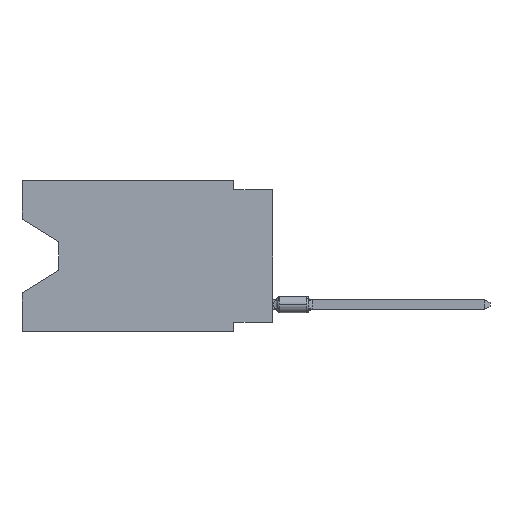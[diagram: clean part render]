
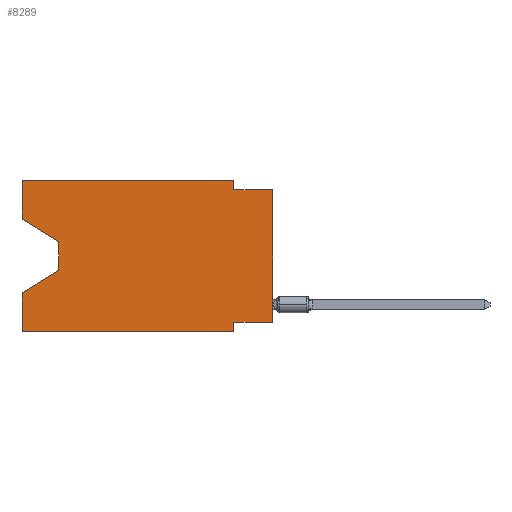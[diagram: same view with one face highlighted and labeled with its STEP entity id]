
A CAD part, left-side view. The second image highlights one B-rep face of the part: STEP entity #8289.
In plain terms, the highlighted planar face has unit normal (-1, 0, 0).
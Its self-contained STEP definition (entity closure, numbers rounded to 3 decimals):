
#38 = EDGE_CURVE ( 'NONE', #6992, #4554, #11585, .T. ) ;
#51 = CARTESIAN_POINT ( 'NONE',  ( 0., 16.383, 0. ) ) ;
#261 = ORIENTED_EDGE ( 'NONE', *, *, #5216, .T. ) ;
#657 = EDGE_CURVE ( 'NONE', #16384, #6992, #19137, .T. ) ;
#970 = CARTESIAN_POINT ( 'NONE',  ( 0., 16.383, 0. ) ) ;
#1034 = DIRECTION ( 'NONE',  ( 0., 0., -1. ) ) ;
#1234 = DIRECTION ( 'NONE',  ( 0., 0., 1. ) ) ;
#1344 = ORIENTED_EDGE ( 'NONE', *, *, #7838, .F. ) ;
#1373 = ORIENTED_EDGE ( 'NONE', *, *, #19129, .F. ) ;
#1385 = VERTEX_POINT ( 'NONE', #15082 ) ;
#1623 = CARTESIAN_POINT ( 'NONE',  ( 0., 13.97, -5.893 ) ) ;
#1732 = DIRECTION ( 'NONE',  ( 0., 0., -1. ) ) ;
#1779 = LINE ( 'NONE', #13912, #6685 ) ;
#2070 = VERTEX_POINT ( 'NONE', #4231 ) ;
#2116 = ORIENTED_EDGE ( 'NONE', *, *, #10446, .T. ) ;
#2195 = CARTESIAN_POINT ( 'NONE',  ( 0., 2.54, -0.635 ) ) ;
#2518 = VECTOR ( 'NONE', #7438, 1000. ) ;
#2958 = EDGE_CURVE ( 'NONE', #16225, #16384, #17965, .T. ) ;
#3040 = CARTESIAN_POINT ( 'NONE',  ( 0., 0., -9.271 ) ) ;
#3101 = VECTOR ( 'NONE', #14318, 1000. ) ;
#3767 = ORIENTED_EDGE ( 'NONE', *, *, #17898, .F. ) ;
#3866 = EDGE_CURVE ( 'NONE', #4252, #8885, #19510, .T. ) ;
#4038 = LINE ( 'NONE', #14684, #13448 ) ;
#4078 = CARTESIAN_POINT ( 'NONE',  ( 0., 16.383, -9.906 ) ) ;
#4117 = CARTESIAN_POINT ( 'NONE',  ( 0., 16.383, 0. ) ) ;
#4231 = CARTESIAN_POINT ( 'NONE',  ( 0., 16.383, -7.36 ) ) ;
#4252 = VERTEX_POINT ( 'NONE', #6393 ) ;
#4554 = VERTEX_POINT ( 'NONE', #18189 ) ;
#5216 = EDGE_CURVE ( 'NONE', #8734, #11478, #4038, .T. ) ;
#6089 = LINE ( 'NONE', #1623, #6399 ) ;
#6177 = VECTOR ( 'NONE', #16123, 1000. ) ;
#6298 = FACE_OUTER_BOUND ( 'NONE', #14487, .T. ) ;
#6393 = CARTESIAN_POINT ( 'NONE',  ( 0., 2.54, -9.271 ) ) ;
#6399 = VECTOR ( 'NONE', #17940, 1000. ) ;
#6685 = VECTOR ( 'NONE', #10828, 1000. ) ;
#6745 = CARTESIAN_POINT ( 'NONE',  ( 0., 0., 0. ) ) ;
#6854 = LINE ( 'NONE', #6745, #3101 ) ;
#6992 = VERTEX_POINT ( 'NONE', #2195 ) ;
#7009 = CARTESIAN_POINT ( 'NONE',  ( 0., 2.54, 0. ) ) ;
#7037 = DIRECTION ( 'NONE',  ( 0., -1., 0. ) ) ;
#7143 = LINE ( 'NONE', #13207, #2518 ) ;
#7438 = DIRECTION ( 'NONE',  ( 0., -1., 0. ) ) ;
#7621 = DIRECTION ( 'NONE',  ( 1., 0., 0. ) ) ;
#7665 = ORIENTED_EDGE ( 'NONE', *, *, #18013, .T. ) ;
#7725 = VECTOR ( 'NONE', #15969, 1000. ) ;
#7838 = EDGE_CURVE ( 'NONE', #10414, #2070, #8766, .T. ) ;
#8057 = ORIENTED_EDGE ( 'NONE', *, *, #38, .F. ) ;
#8289 = ADVANCED_FACE ( 'NONE', ( #6298 ), #13767, .F. ) ;
#8661 = ORIENTED_EDGE ( 'NONE', *, *, #2958, .F. ) ;
#8734 = VERTEX_POINT ( 'NONE', #15611 ) ;
#8766 = LINE ( 'NONE', #17607, #6177 ) ;
#8837 = EDGE_CURVE ( 'NONE', #9446, #4554, #6854, .T. ) ;
#8885 = VERTEX_POINT ( 'NONE', #13509 ) ;
#9446 = VERTEX_POINT ( 'NONE', #3040 ) ;
#9784 = ORIENTED_EDGE ( 'NONE', *, *, #8837, .T. ) ;
#9912 = CARTESIAN_POINT ( 'NONE',  ( 0., 0., -0.635 ) ) ;
#9954 = VECTOR ( 'NONE', #15145, 1000. ) ;
#10137 = DIRECTION ( 'NONE',  ( 0., -0.855, -0.519 ) ) ;
#10298 = VECTOR ( 'NONE', #1034, 1000. ) ;
#10414 = VERTEX_POINT ( 'NONE', #4078 ) ;
#10446 = EDGE_CURVE ( 'NONE', #11478, #1385, #19300, .T. ) ;
#10496 = CARTESIAN_POINT ( 'NONE',  ( 0., 16.383, 0. ) ) ;
#10610 = VECTOR ( 'NONE', #12034, 1000. ) ;
#10828 = DIRECTION ( 'NONE',  ( 0., 1., 0. ) ) ;
#11478 = VERTEX_POINT ( 'NONE', #15258 ) ;
#11585 = LINE ( 'NONE', #9912, #7725 ) ;
#12034 = DIRECTION ( 'NONE',  ( 0., 0., -1. ) ) ;
#12130 = EDGE_CURVE ( 'NONE', #10414, #8885, #7143, .T. ) ;
#12291 = CARTESIAN_POINT ( 'NONE',  ( 0., 2.54, 0. ) ) ;
#13194 = ORIENTED_EDGE ( 'NONE', *, *, #657, .F. ) ;
#13207 = CARTESIAN_POINT ( 'NONE',  ( 0., 16.383, -9.906 ) ) ;
#13448 = VECTOR ( 'NONE', #10137, 1000. ) ;
#13509 = CARTESIAN_POINT ( 'NONE',  ( 0., 2.54, -9.906 ) ) ;
#13742 = CARTESIAN_POINT ( 'NONE',  ( 0., 2.54, -9.906 ) ) ;
#13767 = PLANE ( 'NONE',  #17967 ) ;
#13912 = CARTESIAN_POINT ( 'NONE',  ( 0., 0., -9.271 ) ) ;
#14318 = DIRECTION ( 'NONE',  ( 0., 0., 1. ) ) ;
#14487 = EDGE_LOOP ( 'NONE', ( #261, #2116, #7665, #1344, #15010, #17799, #1373, #9784, #8057, #13194, #8661, #3767 ) ) ;
#14684 = CARTESIAN_POINT ( 'NONE',  ( 0., 16.383, -2.546 ) ) ;
#15010 = ORIENTED_EDGE ( 'NONE', *, *, #12130, .T. ) ;
#15082 = CARTESIAN_POINT ( 'NONE',  ( 0., 13.97, -5.893 ) ) ;
#15145 = DIRECTION ( 'NONE',  ( 0., 0., -1. ) ) ;
#15258 = CARTESIAN_POINT ( 'NONE',  ( 0., 13.97, -4.013 ) ) ;
#15611 = CARTESIAN_POINT ( 'NONE',  ( 0., 16.383, -2.546 ) ) ;
#15619 = VECTOR ( 'NONE', #1234, 1000. ) ;
#15969 = DIRECTION ( 'NONE',  ( 0., -1., 0. ) ) ;
#16123 = DIRECTION ( 'NONE',  ( 0., 0., 1. ) ) ;
#16225 = VERTEX_POINT ( 'NONE', #51 ) ;
#16384 = VERTEX_POINT ( 'NONE', #12291 ) ;
#17607 = CARTESIAN_POINT ( 'NONE',  ( 0., 16.383, 0. ) ) ;
#17750 = LINE ( 'NONE', #4117, #15619 ) ;
#17799 = ORIENTED_EDGE ( 'NONE', *, *, #3866, .F. ) ;
#17898 = EDGE_CURVE ( 'NONE', #8734, #16225, #17750, .T. ) ;
#17940 = DIRECTION ( 'NONE',  ( 0., 0.855, -0.519 ) ) ;
#17965 = LINE ( 'NONE', #970, #18449 ) ;
#17967 = AXIS2_PLACEMENT_3D ( 'NONE', #10496, #7621, #1732 ) ;
#18013 = EDGE_CURVE ( 'NONE', #1385, #2070, #6089, .T. ) ;
#18189 = CARTESIAN_POINT ( 'NONE',  ( 0., 0., -0.635 ) ) ;
#18449 = VECTOR ( 'NONE', #7037, 1000. ) ;
#19129 = EDGE_CURVE ( 'NONE', #9446, #4252, #1779, .T. ) ;
#19137 = LINE ( 'NONE', #7009, #10298 ) ;
#19300 = LINE ( 'NONE', #19482, #10610 ) ;
#19482 = CARTESIAN_POINT ( 'NONE',  ( 0., 13.97, -4.013 ) ) ;
#19510 = LINE ( 'NONE', #13742, #9954 ) ;
